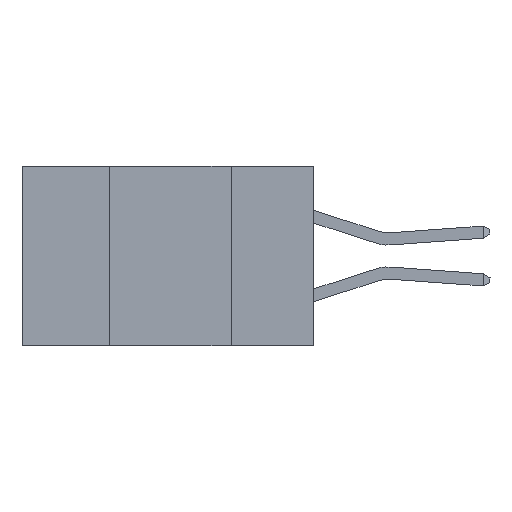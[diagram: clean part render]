
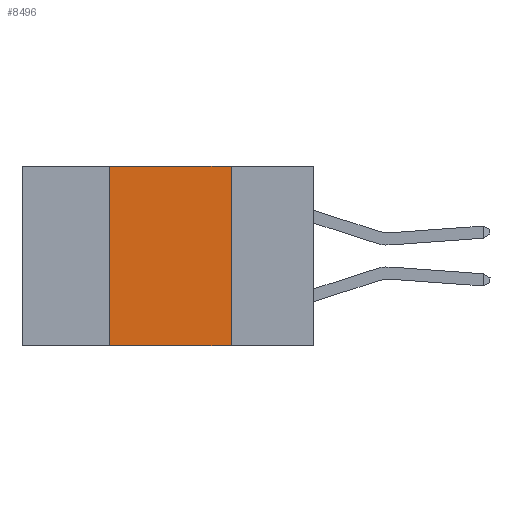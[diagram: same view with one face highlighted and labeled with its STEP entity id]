
A CAD part, left-side view. The second image highlights one B-rep face of the part: STEP entity #8496.
In plain terms, the highlighted planar face has unit normal (-1, 0, 0).
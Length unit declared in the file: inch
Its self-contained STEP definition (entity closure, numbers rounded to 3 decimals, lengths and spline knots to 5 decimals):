
#32 = DIRECTION ( 'NONE',  ( 0., 0., 1. ) ) ;
#45 = DIRECTION ( 'NONE',  ( 0., -1., 0. ) ) ;
#681 = ORIENTED_EDGE ( 'NONE', *, *, #8096, .F. ) ;
#854 = VECTOR ( 'NONE', #12060, 39.37008 ) ;
#1052 = VECTOR ( 'NONE', #8663, 39.37008 ) ;
#1789 = LINE ( 'NONE', #5249, #1052 ) ;
#1945 = CARTESIAN_POINT ( 'NONE',  ( 0., 0.6, -0.37 ) ) ;
#3149 = LINE ( 'NONE', #13441, #9044 ) ;
#3582 = ORIENTED_EDGE ( 'NONE', *, *, #6929, .F. ) ;
#3923 = ORIENTED_EDGE ( 'NONE', *, *, #6766, .F. ) ;
#4082 = LINE ( 'NONE', #8461, #7245 ) ;
#4109 = LINE ( 'NONE', #1945, #854 ) ;
#4827 = PLANE ( 'NONE',  #10643 ) ;
#5249 = CARTESIAN_POINT ( 'NONE',  ( 0., 0.17, 0. ) ) ;
#5279 = CARTESIAN_POINT ( 'NONE',  ( 0., 0.42, -0.37 ) ) ;
#6463 = EDGE_CURVE ( 'NONE', #9407, #8939, #4109, .T. ) ;
#6766 = EDGE_CURVE ( 'NONE', #9407, #7690, #3149, .T. ) ;
#6929 = EDGE_CURVE ( 'NONE', #8289, #8939, #1789, .T. ) ;
#7168 = DIRECTION ( 'NONE',  ( 0., 0., -1. ) ) ;
#7245 = VECTOR ( 'NONE', #45, 39.37008 ) ;
#7673 = CARTESIAN_POINT ( 'NONE',  ( 0., 0.17, 0. ) ) ;
#7690 = VERTEX_POINT ( 'NONE', #10833 ) ;
#8096 = EDGE_CURVE ( 'NONE', #7690, #8289, #4082, .T. ) ;
#8289 = VERTEX_POINT ( 'NONE', #7673 ) ;
#8300 = FACE_OUTER_BOUND ( 'NONE', #12387, .T. ) ;
#8461 = CARTESIAN_POINT ( 'NONE',  ( 0., 0.6, 0. ) ) ;
#8496 = ADVANCED_FACE ( 'NONE', ( #8300 ), #4827, .F. ) ;
#8663 = DIRECTION ( 'NONE',  ( 0., 0., -1. ) ) ;
#8939 = VERTEX_POINT ( 'NONE', #11019 ) ;
#9044 = VECTOR ( 'NONE', #32, 39.37008 ) ;
#9407 = VERTEX_POINT ( 'NONE', #5279 ) ;
#10643 = AXIS2_PLACEMENT_3D ( 'NONE', #12347, #13320, #7168 ) ;
#10833 = CARTESIAN_POINT ( 'NONE',  ( 0., 0.42, 0. ) ) ;
#11019 = CARTESIAN_POINT ( 'NONE',  ( 0., 0.17, -0.37 ) ) ;
#12060 = DIRECTION ( 'NONE',  ( 0., -1., 0. ) ) ;
#12347 = CARTESIAN_POINT ( 'NONE',  ( 0., 0.6, 0. ) ) ;
#12387 = EDGE_LOOP ( 'NONE', ( #3582, #681, #3923, #12945 ) ) ;
#12945 = ORIENTED_EDGE ( 'NONE', *, *, #6463, .T. ) ;
#13320 = DIRECTION ( 'NONE',  ( 1., 0., 0. ) ) ;
#13441 = CARTESIAN_POINT ( 'NONE',  ( 0., 0.42, 0. ) ) ;
